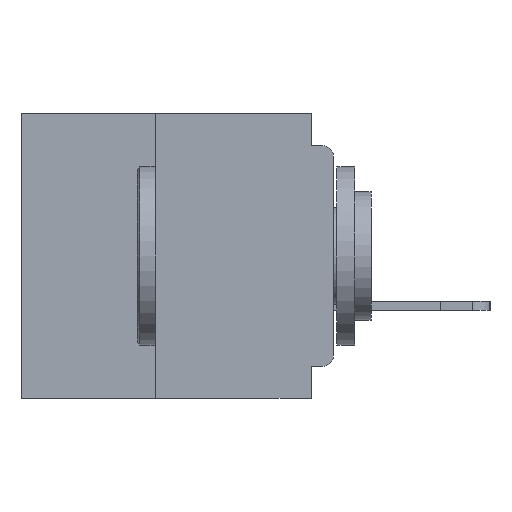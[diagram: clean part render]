
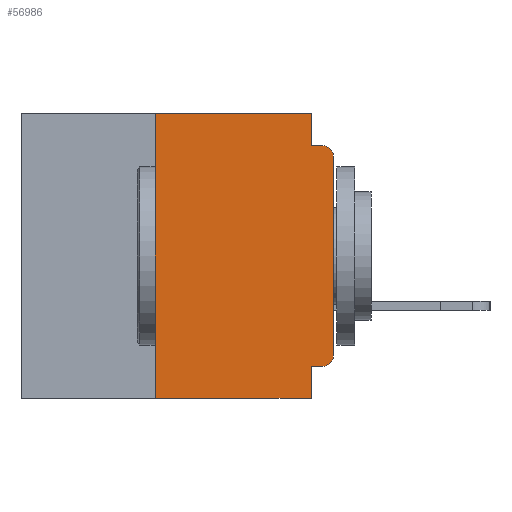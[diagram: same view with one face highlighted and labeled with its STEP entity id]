
A CAD part, left-side view. The second image highlights one B-rep face of the part: STEP entity #56986.
In plain terms, the highlighted planar face has unit normal (-1, 0, 0).
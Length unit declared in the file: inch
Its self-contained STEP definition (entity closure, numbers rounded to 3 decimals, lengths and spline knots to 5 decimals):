
#1302 = EDGE_CURVE ( 'NONE', #55337, #4088, #7163, .T. ) ;
#1757 = LINE ( 'NONE', #45433, #47859 ) ;
#1794 = DIRECTION ( 'NONE',  ( 1., 0., 0. ) ) ;
#2052 = DIRECTION ( 'NONE',  ( -1., 0., 0. ) ) ;
#3060 = EDGE_CURVE ( 'NONE', #13818, #39183, #6941, .T. ) ;
#3852 = ORIENTED_EDGE ( 'NONE', *, *, #17104, .F. ) ;
#4088 = VERTEX_POINT ( 'NONE', #10986 ) ;
#4840 = CARTESIAN_POINT ( 'NONE',  ( 0., 0.015, -0.34 ) ) ;
#5623 = VERTEX_POINT ( 'NONE', #53214 ) ;
#6279 = LINE ( 'NONE', #16523, #28755 ) ;
#6941 = LINE ( 'NONE', #48780, #29408 ) ;
#7163 = LINE ( 'NONE', #27521, #41393 ) ;
#7353 = EDGE_CURVE ( 'NONE', #29348, #5623, #31145, .T. ) ;
#8317 = VERTEX_POINT ( 'NONE', #52494 ) ;
#8789 = CARTESIAN_POINT ( 'NONE',  ( 0., 0., -0.355 ) ) ;
#9056 = VERTEX_POINT ( 'NONE', #30755 ) ;
#9392 = DIRECTION ( 'NONE',  ( 0., 0., -1. ) ) ;
#10558 = CIRCLE ( 'NONE', #19504, 0.015 ) ;
#10737 = LINE ( 'NONE', #12298, #43468 ) ;
#10986 = CARTESIAN_POINT ( 'NONE',  ( 0., 0.031, -0.4 ) ) ;
#11518 = ORIENTED_EDGE ( 'NONE', *, *, #18761, .F. ) ;
#12006 = CARTESIAN_POINT ( 'NONE',  ( 0., 0., -0.34 ) ) ;
#12092 = ORIENTED_EDGE ( 'NONE', *, *, #18940, .F. ) ;
#12298 = CARTESIAN_POINT ( 'NONE',  ( 0., 0.25, -0.4 ) ) ;
#13818 = VERTEX_POINT ( 'NONE', #12006 ) ;
#14366 = CARTESIAN_POINT ( 'NONE',  ( 0., 0.031, -0.045 ) ) ;
#14729 = ORIENTED_EDGE ( 'NONE', *, *, #42375, .T. ) ;
#15664 = AXIS2_PLACEMENT_3D ( 'NONE', #46322, #1794, #33189 ) ;
#16523 = CARTESIAN_POINT ( 'NONE',  ( 0., 0.437, 0. ) ) ;
#17104 = EDGE_CURVE ( 'NONE', #41689, #9056, #1757, .T. ) ;
#18390 = CARTESIAN_POINT ( 'NONE',  ( 0., 0., -0.06 ) ) ;
#18761 = EDGE_CURVE ( 'NONE', #8317, #41689, #41436, .T. ) ;
#18940 = EDGE_CURVE ( 'NONE', #55337, #50811, #10737, .T. ) ;
#19504 = AXIS2_PLACEMENT_3D ( 'NONE', #29004, #2052, #33427 ) ;
#20365 = CARTESIAN_POINT ( 'NONE',  ( 0., 0.25, -0.4 ) ) ;
#21462 = EDGE_CURVE ( 'NONE', #50811, #8317, #6279, .T. ) ;
#22032 = EDGE_LOOP ( 'NONE', ( #46597, #14729, #3852, #11518, #28501, #12092, #48779, #26875, #44976, #56338 ) ) ;
#23963 = CARTESIAN_POINT ( 'NONE',  ( 0., 0.031, 0. ) ) ;
#26167 = FACE_OUTER_BOUND ( 'NONE', #22032, .T. ) ;
#26495 = DIRECTION ( 'NONE',  ( 0., -1., 0. ) ) ;
#26875 = ORIENTED_EDGE ( 'NONE', *, *, #34689, .F. ) ;
#27521 = CARTESIAN_POINT ( 'NONE',  ( 0., 0.437, -0.4 ) ) ;
#27804 = LINE ( 'NONE', #53998, #49903 ) ;
#28501 = ORIENTED_EDGE ( 'NONE', *, *, #21462, .F. ) ;
#28539 = PLANE ( 'NONE',  #15664 ) ;
#28755 = VECTOR ( 'NONE', #38880, 39.37008 ) ;
#29004 = CARTESIAN_POINT ( 'NONE',  ( 0., 0.015, -0.06 ) ) ;
#29348 = VERTEX_POINT ( 'NONE', #41818 ) ;
#29408 = VECTOR ( 'NONE', #48287, 39.37008 ) ;
#29674 = VECTOR ( 'NONE', #54872, 39.37008 ) ;
#29754 = VECTOR ( 'NONE', #48891, 39.37008 ) ;
#30755 = CARTESIAN_POINT ( 'NONE',  ( 0., 0.015, -0.045 ) ) ;
#31145 = LINE ( 'NONE', #8789, #29754 ) ;
#33189 = DIRECTION ( 'NONE',  ( 0., 0., -1. ) ) ;
#33427 = DIRECTION ( 'NONE',  ( 0., 0., -1. ) ) ;
#34689 = EDGE_CURVE ( 'NONE', #5623, #4088, #27804, .T. ) ;
#34740 = DIRECTION ( 'NONE',  ( 0., 0., 1. ) ) ;
#36137 = DIRECTION ( 'NONE',  ( -1., 0., 0. ) ) ;
#36426 = DIRECTION ( 'NONE',  ( 0., 0., -1. ) ) ;
#38557 = EDGE_CURVE ( 'NONE', #29348, #13818, #48807, .T. ) ;
#38880 = DIRECTION ( 'NONE',  ( 0., -1., 0. ) ) ;
#39183 = VERTEX_POINT ( 'NONE', #18390 ) ;
#41009 = DIRECTION ( 'NONE',  ( 0., -1., 0. ) ) ;
#41393 = VECTOR ( 'NONE', #26495, 39.37008 ) ;
#41436 = LINE ( 'NONE', #23963, #29674 ) ;
#41555 = CARTESIAN_POINT ( 'NONE',  ( 0., 0.25, 0. ) ) ;
#41689 = VERTEX_POINT ( 'NONE', #14366 ) ;
#41818 = CARTESIAN_POINT ( 'NONE',  ( 0., 0.015, -0.355 ) ) ;
#42375 = EDGE_CURVE ( 'NONE', #39183, #9056, #10558, .T. ) ;
#43468 = VECTOR ( 'NONE', #34740, 39.37008 ) ;
#44976 = ORIENTED_EDGE ( 'NONE', *, *, #7353, .F. ) ;
#45433 = CARTESIAN_POINT ( 'NONE',  ( 0., 0., -0.045 ) ) ;
#46322 = CARTESIAN_POINT ( 'NONE',  ( 0., 0.437, 0. ) ) ;
#46597 = ORIENTED_EDGE ( 'NONE', *, *, #3060, .T. ) ;
#47859 = VECTOR ( 'NONE', #41009, 39.37008 ) ;
#48287 = DIRECTION ( 'NONE',  ( 0., 0., 1. ) ) ;
#48779 = ORIENTED_EDGE ( 'NONE', *, *, #1302, .T. ) ;
#48780 = CARTESIAN_POINT ( 'NONE',  ( 0., 0., 0. ) ) ;
#48807 = CIRCLE ( 'NONE', #56578, 0.015 ) ;
#48891 = DIRECTION ( 'NONE',  ( 0., 1., 0. ) ) ;
#49903 = VECTOR ( 'NONE', #36426, 39.37008 ) ;
#50811 = VERTEX_POINT ( 'NONE', #41555 ) ;
#52494 = CARTESIAN_POINT ( 'NONE',  ( 0., 0.031, 0. ) ) ;
#53214 = CARTESIAN_POINT ( 'NONE',  ( 0., 0.031, -0.355 ) ) ;
#53998 = CARTESIAN_POINT ( 'NONE',  ( 0., 0.031, -0.4 ) ) ;
#54872 = DIRECTION ( 'NONE',  ( 0., 0., -1. ) ) ;
#55337 = VERTEX_POINT ( 'NONE', #20365 ) ;
#56338 = ORIENTED_EDGE ( 'NONE', *, *, #38557, .T. ) ;
#56578 = AXIS2_PLACEMENT_3D ( 'NONE', #4840, #36137, #9392 ) ;
#56986 = ADVANCED_FACE ( 'NONE', ( #26167 ), #28539, .F. ) ;
